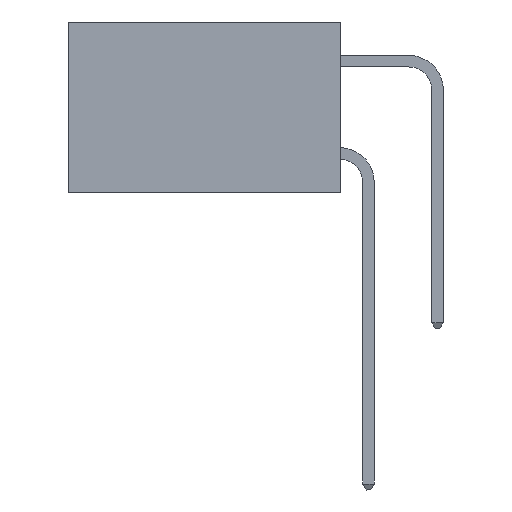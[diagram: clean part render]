
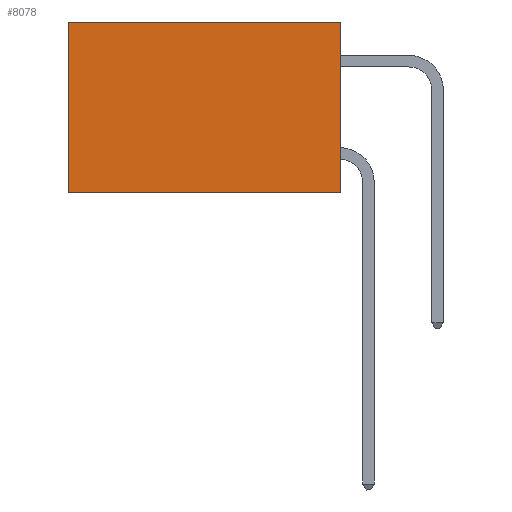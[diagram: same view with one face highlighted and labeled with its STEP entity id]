
A CAD part, left-side view. The second image highlights one B-rep face of the part: STEP entity #8078.
In plain terms, the highlighted planar face has unit normal (-1, 0, 0).
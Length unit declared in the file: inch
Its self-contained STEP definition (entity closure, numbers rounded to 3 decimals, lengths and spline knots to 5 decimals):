
#321 = EDGE_LOOP ( 'NONE', ( #9717, #5496, #5338, #6104 ) ) ;
#386 = DIRECTION ( 'NONE',  ( 1., 0., 0. ) ) ;
#531 = VECTOR ( 'NONE', #1861, 39.37008 ) ;
#571 = DIRECTION ( 'NONE',  ( 0., 1., 0. ) ) ;
#700 = VECTOR ( 'NONE', #12915, 39.37008 ) ;
#1861 = DIRECTION ( 'NONE',  ( 0., 0., -1. ) ) ;
#2212 = FACE_OUTER_BOUND ( 'NONE', #321, .T. ) ;
#2388 = LINE ( 'NONE', #7894, #6806 ) ;
#2453 = CARTESIAN_POINT ( 'NONE',  ( 0.277, 0.59, 0. ) ) ;
#3953 = EDGE_CURVE ( 'NONE', #12008, #8989, #12482, .T. ) ;
#4177 = AXIS2_PLACEMENT_3D ( 'NONE', #4837, #386, #10778 ) ;
#4837 = CARTESIAN_POINT ( 'NONE',  ( 0.277, 0., -0.37 ) ) ;
#5338 = ORIENTED_EDGE ( 'NONE', *, *, #3953, .F. ) ;
#5496 = ORIENTED_EDGE ( 'NONE', *, *, #12071, .F. ) ;
#6104 = ORIENTED_EDGE ( 'NONE', *, *, #9835, .T. ) ;
#6377 = CARTESIAN_POINT ( 'NONE',  ( 0.277, 0., 0. ) ) ;
#6806 = VECTOR ( 'NONE', #17768, 39.37008 ) ;
#7536 = CARTESIAN_POINT ( 'NONE',  ( 0.277, 0., -0.37 ) ) ;
#7744 = PLANE ( 'NONE',  #4177 ) ;
#7894 = CARTESIAN_POINT ( 'NONE',  ( 0.277, 0., 0. ) ) ;
#8078 = ADVANCED_FACE ( 'NONE', ( #2212 ), #7744, .F. ) ;
#8989 = VERTEX_POINT ( 'NONE', #7536 ) ;
#9717 = ORIENTED_EDGE ( 'NONE', *, *, #15880, .T. ) ;
#9835 = EDGE_CURVE ( 'NONE', #12008, #12907, #2388, .T. ) ;
#10715 = CARTESIAN_POINT ( 'NONE',  ( 0.277, 0.59, -0.37 ) ) ;
#10778 = DIRECTION ( 'NONE',  ( 0., 0., -1. ) ) ;
#11867 = LINE ( 'NONE', #10715, #531 ) ;
#12008 = VERTEX_POINT ( 'NONE', #6377 ) ;
#12071 = EDGE_CURVE ( 'NONE', #8989, #12100, #12867, .T. ) ;
#12100 = VERTEX_POINT ( 'NONE', #17907 ) ;
#12401 = CARTESIAN_POINT ( 'NONE',  ( 0.277, 0., -0.37 ) ) ;
#12422 = VECTOR ( 'NONE', #571, 39.37008 ) ;
#12482 = LINE ( 'NONE', #12543, #700 ) ;
#12543 = CARTESIAN_POINT ( 'NONE',  ( 0.277, 0., -0.37 ) ) ;
#12867 = LINE ( 'NONE', #12401, #12422 ) ;
#12907 = VERTEX_POINT ( 'NONE', #2453 ) ;
#12915 = DIRECTION ( 'NONE',  ( 0., 0., -1. ) ) ;
#15880 = EDGE_CURVE ( 'NONE', #12907, #12100, #11867, .T. ) ;
#17768 = DIRECTION ( 'NONE',  ( 0., 1., 0. ) ) ;
#17907 = CARTESIAN_POINT ( 'NONE',  ( 0.277, 0.59, -0.37 ) ) ;
